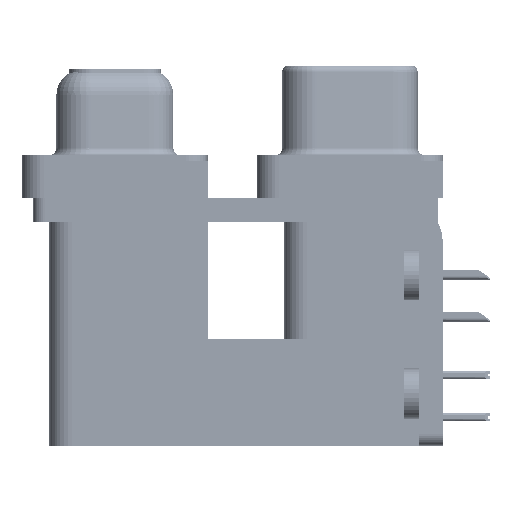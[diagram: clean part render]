
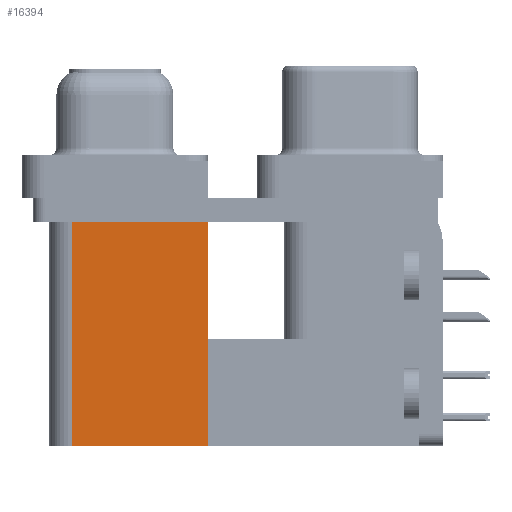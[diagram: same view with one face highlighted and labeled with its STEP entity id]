
A CAD part, left-side view. The second image highlights one B-rep face of the part: STEP entity #16394.
In plain terms, the highlighted planar face has unit normal (-1, 0, 0).
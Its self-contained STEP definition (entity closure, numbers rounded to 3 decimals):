
#2169 = ORIENTED_EDGE ( 'NONE', *, *, #33155, .T. ) ;
#2250 = DIRECTION ( 'NONE',  ( 0., 0., 1. ) ) ;
#4283 = DIRECTION ( 'NONE',  ( 0., 1., 0. ) ) ;
#6080 = DIRECTION ( 'NONE',  ( 0., 0., 1. ) ) ;
#6639 = FACE_OUTER_BOUND ( 'NONE', #50588, .T. ) ;
#7568 = CARTESIAN_POINT ( 'NONE',  ( 3.79, 18.8, -19.2 ) ) ;
#8995 = CARTESIAN_POINT ( 'NONE',  ( 3.79, 18.8, -19.2 ) ) ;
#9611 = LINE ( 'NONE', #31227, #13141 ) ;
#12445 = VERTEX_POINT ( 'NONE', #46417 ) ;
#12532 = VECTOR ( 'NONE', #52112, 1000. ) ;
#13141 = VECTOR ( 'NONE', #4283, 1000. ) ;
#16394 = ADVANCED_FACE ( 'NONE', ( #6639 ), #61617, .F. ) ;
#16685 = LINE ( 'NONE', #21652, #59680 ) ;
#19163 = VERTEX_POINT ( 'NONE', #8995 ) ;
#20166 = LINE ( 'NONE', #30487, #12532 ) ;
#21652 = CARTESIAN_POINT ( 'NONE',  ( 3.79, 9.6, -19.2 ) ) ;
#28481 = LINE ( 'NONE', #7568, #62712 ) ;
#30487 = CARTESIAN_POINT ( 'NONE',  ( 3.79, 9.6, -19.2 ) ) ;
#31227 = CARTESIAN_POINT ( 'NONE',  ( 3.79, 9.6, -2.5 ) ) ;
#33155 = EDGE_CURVE ( 'NONE', #12445, #34099, #9611, .T. ) ;
#34099 = VERTEX_POINT ( 'NONE', #38854 ) ;
#37043 = ORIENTED_EDGE ( 'NONE', *, *, #63522, .T. ) ;
#38854 = CARTESIAN_POINT ( 'NONE',  ( 3.79, 18.8, -2.5 ) ) ;
#39607 = DIRECTION ( 'NONE',  ( 1., 0., 0. ) ) ;
#40041 = EDGE_CURVE ( 'NONE', #54230, #19163, #20166, .T. ) ;
#46417 = CARTESIAN_POINT ( 'NONE',  ( 3.79, 9.6, -2.5 ) ) ;
#49841 = AXIS2_PLACEMENT_3D ( 'NONE', #55204, #39607, #49890 ) ;
#49890 = DIRECTION ( 'NONE',  ( 0., 1., 0. ) ) ;
#50588 = EDGE_LOOP ( 'NONE', ( #2169, #55620, #56201, #37043 ) ) ;
#52112 = DIRECTION ( 'NONE',  ( 0., 1., 0. ) ) ;
#54230 = VERTEX_POINT ( 'NONE', #64958 ) ;
#55204 = CARTESIAN_POINT ( 'NONE',  ( 3.79, 9.6, -19.2 ) ) ;
#55620 = ORIENTED_EDGE ( 'NONE', *, *, #57969, .F. ) ;
#56201 = ORIENTED_EDGE ( 'NONE', *, *, #40041, .F. ) ;
#57969 = EDGE_CURVE ( 'NONE', #19163, #34099, #28481, .T. ) ;
#59680 = VECTOR ( 'NONE', #6080, 1000. ) ;
#61617 = PLANE ( 'NONE',  #49841 ) ;
#62712 = VECTOR ( 'NONE', #2250, 1000. ) ;
#63522 = EDGE_CURVE ( 'NONE', #54230, #12445, #16685, .T. ) ;
#64958 = CARTESIAN_POINT ( 'NONE',  ( 3.79, 9.6, -19.2 ) ) ;
